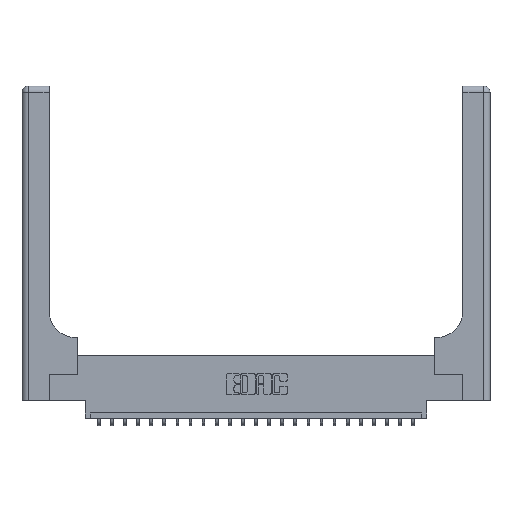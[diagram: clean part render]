
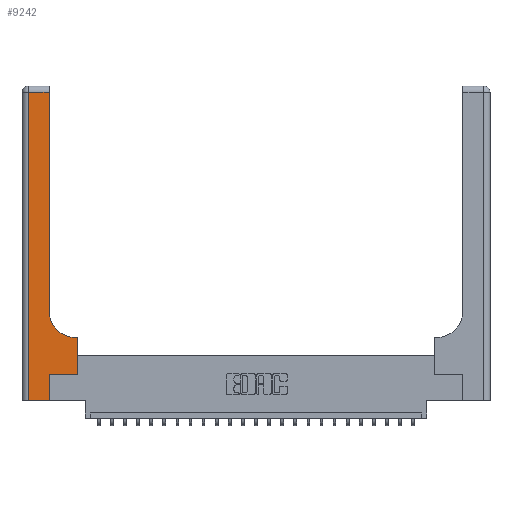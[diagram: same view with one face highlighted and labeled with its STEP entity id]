
A CAD part, top view. The second image highlights one B-rep face of the part: STEP entity #9242.
In plain terms, the highlighted planar face has unit normal (0, 0, 1).
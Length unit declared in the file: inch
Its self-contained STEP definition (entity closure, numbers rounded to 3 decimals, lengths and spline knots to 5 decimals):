
#157 = VECTOR ( 'NONE', #8542, 39.37008 ) ;
#224 = DIRECTION ( 'NONE',  ( -1., 0., 0. ) ) ;
#558 = EDGE_CURVE ( 'NONE', #818, #1120, #2873, .T. ) ;
#818 = VERTEX_POINT ( 'NONE', #7619 ) ;
#1120 = VERTEX_POINT ( 'NONE', #18333 ) ;
#1535 = DIRECTION ( 'NONE',  ( 0., 0., -1. ) ) ;
#1583 = VERTEX_POINT ( 'NONE', #17703 ) ;
#1650 = PLANE ( 'NONE',  #18252 ) ;
#1666 = EDGE_CURVE ( 'NONE', #1583, #15240, #13214, .T. ) ;
#2436 = CIRCLE ( 'NONE', #5230, 0.25 ) ;
#2483 = CARTESIAN_POINT ( 'NONE',  ( 0.06, 0., 0.37 ) ) ;
#2584 = VECTOR ( 'NONE', #22243, 39.37008 ) ;
#2873 = LINE ( 'NONE', #22914, #16610 ) ;
#2945 = CARTESIAN_POINT ( 'NONE',  ( 0.06, 3., 0.37 ) ) ;
#3159 = LINE ( 'NONE', #6242, #2584 ) ;
#3160 = VERTEX_POINT ( 'NONE', #17552 ) ;
#3361 = VERTEX_POINT ( 'NONE', #11044 ) ;
#3547 = ORIENTED_EDGE ( 'NONE', *, *, #10783, .T. ) ;
#4249 = EDGE_CURVE ( 'NONE', #3361, #16309, #10324, .T. ) ;
#4339 = ORIENTED_EDGE ( 'NONE', *, *, #22645, .T. ) ;
#4721 = EDGE_CURVE ( 'NONE', #15240, #19895, #19513, .T. ) ;
#5230 = AXIS2_PLACEMENT_3D ( 'NONE', #12305, #1535, #14105 ) ;
#5277 = DIRECTION ( 'NONE',  ( -1., 0., 0. ) ) ;
#5319 = DIRECTION ( 'NONE',  ( 0., 1., 0. ) ) ;
#5603 = CARTESIAN_POINT ( 'NONE',  ( 0., 2.94, 0.37 ) ) ;
#5768 = ORIENTED_EDGE ( 'NONE', *, *, #12080, .T. ) ;
#6242 = CARTESIAN_POINT ( 'NONE',  ( 0., 0., 0.37 ) ) ;
#6492 = DIRECTION ( 'NONE',  ( 0., -1., 0. ) ) ;
#6990 = CARTESIAN_POINT ( 'NONE',  ( 0.528, 0.25, 0.37 ) ) ;
#7619 = CARTESIAN_POINT ( 'NONE',  ( 0.265, 0.25, 0.37 ) ) ;
#7872 = VECTOR ( 'NONE', #12018, 39.37008 ) ;
#8542 = DIRECTION ( 'NONE',  ( -1., 0., 0. ) ) ;
#9242 = ADVANCED_FACE ( 'NONE', ( #11798 ), #1650, .F. ) ;
#9301 = VECTOR ( 'NONE', #5319, 39.37008 ) ;
#9499 = CARTESIAN_POINT ( 'NONE',  ( 0.51, 0.6, 0.37 ) ) ;
#9863 = LINE ( 'NONE', #19625, #9301 ) ;
#10324 = LINE ( 'NONE', #19220, #157 ) ;
#10665 = CARTESIAN_POINT ( 'NONE',  ( 0.26, 0.85, 0.37 ) ) ;
#10783 = EDGE_CURVE ( 'NONE', #16309, #16686, #2436, .T. ) ;
#11044 = CARTESIAN_POINT ( 'NONE',  ( 0.528, 0.6, 0.37 ) ) ;
#11337 = ORIENTED_EDGE ( 'NONE', *, *, #4249, .T. ) ;
#11798 = FACE_OUTER_BOUND ( 'NONE', #12304, .T. ) ;
#12018 = DIRECTION ( 'NONE',  ( 0., 1., 0. ) ) ;
#12080 = EDGE_CURVE ( 'NONE', #1120, #3361, #13084, .T. ) ;
#12304 = EDGE_LOOP ( 'NONE', ( #17399, #13785, #16304, #19846, #4339, #12725, #5768, #11337, #3547 ) ) ;
#12305 = CARTESIAN_POINT ( 'NONE',  ( 0.51, 0.85, 0.37 ) ) ;
#12725 = ORIENTED_EDGE ( 'NONE', *, *, #558, .T. ) ;
#13084 = LINE ( 'NONE', #6990, #22548 ) ;
#13214 = LINE ( 'NONE', #5603, #13769 ) ;
#13769 = VECTOR ( 'NONE', #224, 39.37008 ) ;
#13785 = ORIENTED_EDGE ( 'NONE', *, *, #1666, .T. ) ;
#14105 = DIRECTION ( 'NONE',  ( 1., 0., 0. ) ) ;
#14226 = CARTESIAN_POINT ( 'NONE',  ( 0., 3., 0.37 ) ) ;
#15240 = VERTEX_POINT ( 'NONE', #21828 ) ;
#16002 = DIRECTION ( 'NONE',  ( 0., 0., -1. ) ) ;
#16304 = ORIENTED_EDGE ( 'NONE', *, *, #4721, .T. ) ;
#16309 = VERTEX_POINT ( 'NONE', #9499 ) ;
#16610 = VECTOR ( 'NONE', #17602, 39.37008 ) ;
#16686 = VERTEX_POINT ( 'NONE', #10665 ) ;
#17399 = ORIENTED_EDGE ( 'NONE', *, *, #22796, .T. ) ;
#17552 = CARTESIAN_POINT ( 'NONE',  ( 0.265, 0., 0.37 ) ) ;
#17602 = DIRECTION ( 'NONE',  ( 1., 0., 0. ) ) ;
#17703 = CARTESIAN_POINT ( 'NONE',  ( 0.26, 2.94, 0.37 ) ) ;
#18252 = AXIS2_PLACEMENT_3D ( 'NONE', #14226, #16002, #5277 ) ;
#18333 = CARTESIAN_POINT ( 'NONE',  ( 0.528, 0.25, 0.37 ) ) ;
#18938 = VECTOR ( 'NONE', #6492, 39.37008 ) ;
#19220 = CARTESIAN_POINT ( 'NONE',  ( 0.26, 0.6, 0.37 ) ) ;
#19470 = DIRECTION ( 'NONE',  ( 0., 1., 0. ) ) ;
#19513 = LINE ( 'NONE', #2945, #18938 ) ;
#19625 = CARTESIAN_POINT ( 'NONE',  ( 0.26, 3., 0.37 ) ) ;
#19846 = ORIENTED_EDGE ( 'NONE', *, *, #20529, .T. ) ;
#19895 = VERTEX_POINT ( 'NONE', #2483 ) ;
#20529 = EDGE_CURVE ( 'NONE', #19895, #3160, #3159, .T. ) ;
#20804 = CARTESIAN_POINT ( 'NONE',  ( 0.265, 0., 0.37 ) ) ;
#21828 = CARTESIAN_POINT ( 'NONE',  ( 0.06, 2.94, 0.37 ) ) ;
#22111 = LINE ( 'NONE', #20804, #7872 ) ;
#22243 = DIRECTION ( 'NONE',  ( 1., 0., 0. ) ) ;
#22548 = VECTOR ( 'NONE', #19470, 39.37008 ) ;
#22645 = EDGE_CURVE ( 'NONE', #3160, #818, #22111, .T. ) ;
#22796 = EDGE_CURVE ( 'NONE', #16686, #1583, #9863, .T. ) ;
#22914 = CARTESIAN_POINT ( 'NONE',  ( 0.265, 0.25, 0.37 ) ) ;
